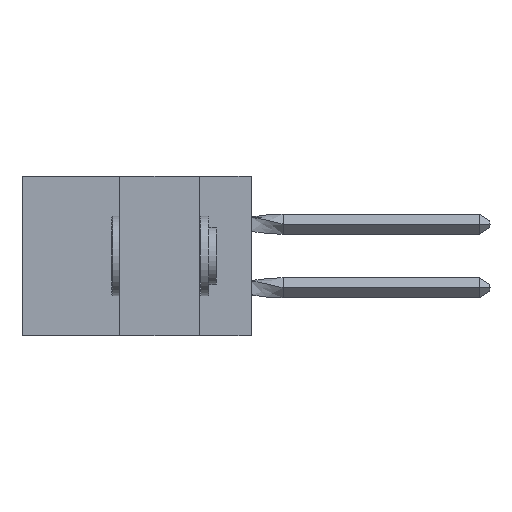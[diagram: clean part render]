
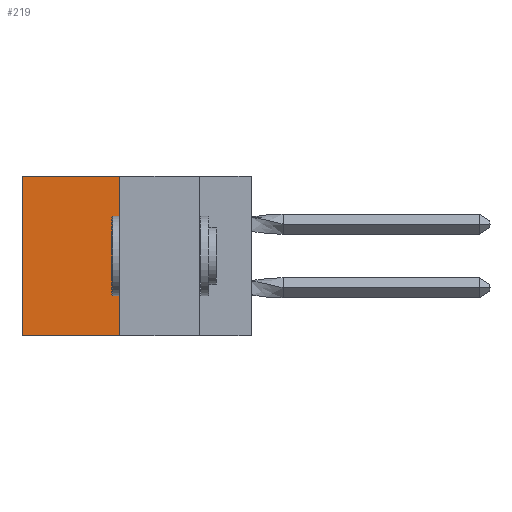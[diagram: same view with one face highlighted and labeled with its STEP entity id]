
A CAD part, left-side view. The second image highlights one B-rep face of the part: STEP entity #219.
In plain terms, the highlighted planar face has unit normal (-1, 0, 0).
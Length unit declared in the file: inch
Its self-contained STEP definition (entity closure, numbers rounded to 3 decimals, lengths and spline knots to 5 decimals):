
#137 = ORIENTED_EDGE ( 'NONE', *, *, #10896, .T. ) ;
#142 = VECTOR ( 'NONE', #11496, 39.37008 ) ;
#219 = ADVANCED_FACE ( 'NONE', ( #13917 ), #593, .F. ) ;
#593 = PLANE ( 'NONE',  #11341 ) ;
#863 = CARTESIAN_POINT ( 'NONE',  ( 0.305, 0.413, -0.5 ) ) ;
#1245 = DIRECTION ( 'NONE',  ( 0., 1., 0. ) ) ;
#1275 = EDGE_CURVE ( 'NONE', #11283, #2211, #2898, .T. ) ;
#1420 = VECTOR ( 'NONE', #4285, 39.37008 ) ;
#2211 = VERTEX_POINT ( 'NONE', #7345 ) ;
#2471 = ORIENTED_EDGE ( 'NONE', *, *, #1275, .T. ) ;
#2898 = LINE ( 'NONE', #6609, #4503 ) ;
#4285 = DIRECTION ( 'NONE',  ( 0., 0., -1. ) ) ;
#4503 = VECTOR ( 'NONE', #6697, 39.37008 ) ;
#5014 = EDGE_CURVE ( 'NONE', #10083, #2211, #7898, .T. ) ;
#6234 = CARTESIAN_POINT ( 'NONE',  ( 0.305, 0.413, -0.5 ) ) ;
#6609 = CARTESIAN_POINT ( 'NONE',  ( 0.305, 0.72, -0.5 ) ) ;
#6697 = DIRECTION ( 'NONE',  ( 0., 0., -1. ) ) ;
#6816 = ORIENTED_EDGE ( 'NONE', *, *, #5014, .F. ) ;
#7345 = CARTESIAN_POINT ( 'NONE',  ( 0.305, 0.72, -0.5 ) ) ;
#7546 = CARTESIAN_POINT ( 'NONE',  ( 0.305, 0.72, 0. ) ) ;
#7664 = ORIENTED_EDGE ( 'NONE', *, *, #11360, .F. ) ;
#7887 = CARTESIAN_POINT ( 'NONE',  ( 0.305, 0.413, 0. ) ) ;
#7898 = LINE ( 'NONE', #8049, #11982 ) ;
#8049 = CARTESIAN_POINT ( 'NONE',  ( 0.305, 0.413, -0.5 ) ) ;
#8890 = EDGE_LOOP ( 'NONE', ( #2471, #6816, #7664, #137 ) ) ;
#8986 = CARTESIAN_POINT ( 'NONE',  ( 0.305, 0.413, 0. ) ) ;
#10083 = VERTEX_POINT ( 'NONE', #13314 ) ;
#10896 = EDGE_CURVE ( 'NONE', #12663, #11283, #11276, .T. ) ;
#11276 = LINE ( 'NONE', #7887, #142 ) ;
#11283 = VERTEX_POINT ( 'NONE', #7546 ) ;
#11341 = AXIS2_PLACEMENT_3D ( 'NONE', #6234, #13974, #12869 ) ;
#11360 = EDGE_CURVE ( 'NONE', #12663, #10083, #14007, .T. ) ;
#11496 = DIRECTION ( 'NONE',  ( 0., 1., 0. ) ) ;
#11982 = VECTOR ( 'NONE', #1245, 39.37008 ) ;
#12663 = VERTEX_POINT ( 'NONE', #8986 ) ;
#12869 = DIRECTION ( 'NONE',  ( 0., 0., -1. ) ) ;
#13314 = CARTESIAN_POINT ( 'NONE',  ( 0.305, 0.413, -0.5 ) ) ;
#13917 = FACE_OUTER_BOUND ( 'NONE', #8890, .T. ) ;
#13974 = DIRECTION ( 'NONE',  ( 1., 0., 0. ) ) ;
#14007 = LINE ( 'NONE', #863, #1420 ) ;
